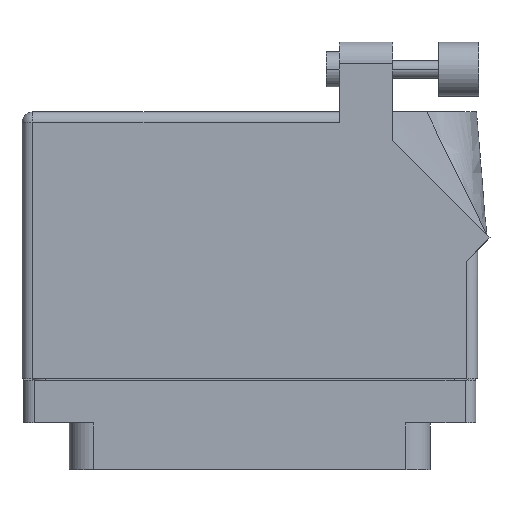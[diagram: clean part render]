
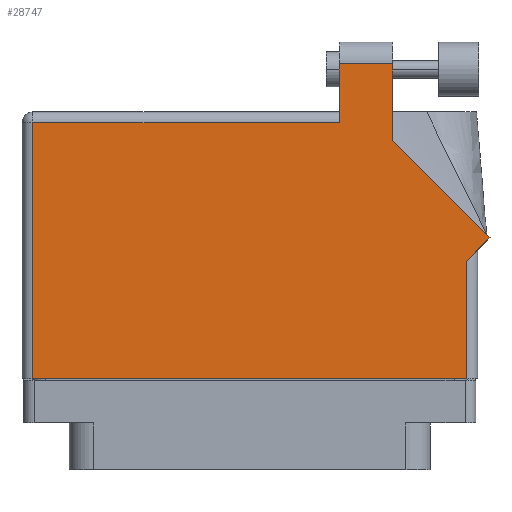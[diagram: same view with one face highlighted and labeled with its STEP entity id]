
A CAD part, front view. The second image highlights one B-rep face of the part: STEP entity #28747.
In plain terms, the highlighted face is planar.
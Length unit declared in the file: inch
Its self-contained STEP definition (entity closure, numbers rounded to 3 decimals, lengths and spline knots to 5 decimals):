
#9 = CARTESIAN_POINT ( 'NONE',  ( -1.306, -0.1, 0.455 ) ) ;
#409 = DIRECTION ( 'NONE',  ( 0., 0., -1. ) ) ;
#1162 = CARTESIAN_POINT ( 'NONE',  ( 1.37671, 0.70771, 0.455 ) ) ;
#1805 = EDGE_CURVE ( 'NONE', #40076, #41135, #41123, .T. ) ;
#1938 = LINE ( 'NONE', #38785, #34554 ) ;
#2650 = ORIENTED_EDGE ( 'NONE', *, *, #43815, .T. ) ;
#3377 = DIRECTION ( 'NONE',  ( -1., 0., 0. ) ) ;
#4816 = EDGE_CURVE ( 'NONE', #47818, #17974, #12187, .T. ) ;
#4828 = EDGE_CURVE ( 'NONE', #51017, #42544, #13381, .T. ) ;
#5143 = CARTESIAN_POINT ( 'NONE',  ( -1.306, 1.43, 0.455 ) ) ;
#5159 = LINE ( 'NONE', #15454, #8283 ) ;
#5259 = VECTOR ( 'NONE', #15422, 39.37008 ) ;
#7045 = CARTESIAN_POINT ( 'NONE',  ( 0.513, 1.705, 0.455 ) ) ;
#7877 = CARTESIAN_POINT ( 'NONE',  ( 0.82, 1.26442, 0.455 ) ) ;
#7932 = ORIENTED_EDGE ( 'NONE', *, *, #10526, .T. ) ;
#8283 = VECTOR ( 'NONE', #3377, 39.37008 ) ;
#10526 = EDGE_CURVE ( 'NONE', #32718, #30651, #5159, .T. ) ;
#11070 = VERTEX_POINT ( 'NONE', #44175 ) ;
#11456 = DIRECTION ( 'NONE',  ( 0., -1., 0. ) ) ;
#11790 = LINE ( 'NONE', #23769, #35677 ) ;
#12187 = LINE ( 'NONE', #9, #34750 ) ;
#12846 = PLANE ( 'NONE',  #20259 ) ;
#13381 = LINE ( 'NONE', #32285, #5259 ) ;
#14507 = DIRECTION ( 'NONE',  ( 0., 1., 0. ) ) ;
#15422 = DIRECTION ( 'NONE',  ( -0.707, 0.707, 0. ) ) ;
#15454 = CARTESIAN_POINT ( 'NONE',  ( 0.513, 1.705, 0.455 ) ) ;
#17049 = LINE ( 'NONE', #35463, #17657 ) ;
#17657 = VECTOR ( 'NONE', #11456, 39.37008 ) ;
#17974 = VERTEX_POINT ( 'NONE', #19095 ) ;
#18078 = ORIENTED_EDGE ( 'NONE', *, *, #4816, .T. ) ;
#19095 = CARTESIAN_POINT ( 'NONE',  ( 1.244, -0.1, 0.455 ) ) ;
#19635 = DIRECTION ( 'NONE',  ( 1., 0., 0. ) ) ;
#19949 = ORIENTED_EDGE ( 'NONE', *, *, #25836, .T. ) ;
#20259 = AXIS2_PLACEMENT_3D ( 'NONE', #5143, #409, #45152 ) ;
#21161 = LINE ( 'NONE', #22234, #22426 ) ;
#22234 = CARTESIAN_POINT ( 'NONE',  ( 1.244, 0.637, 0.455 ) ) ;
#22426 = VECTOR ( 'NONE', #14507, 39.37008 ) ;
#23164 = EDGE_LOOP ( 'NONE', ( #2650, #7932, #44292, #31699, #47061, #18078, #32034, #19949, #40817 ) ) ;
#23464 = DIRECTION ( 'NONE',  ( 0., 1., 0. ) ) ;
#23769 = CARTESIAN_POINT ( 'NONE',  ( 1.306, 0.637, 0.455 ) ) ;
#24046 = CARTESIAN_POINT ( 'NONE',  ( 0.82, 1.705, 0.455 ) ) ;
#24895 = CARTESIAN_POINT ( 'NONE',  ( -1.244, 1.368, 0.455 ) ) ;
#25836 = EDGE_CURVE ( 'NONE', #11070, #51017, #11790, .T. ) ;
#27938 = EDGE_CURVE ( 'NONE', #30651, #40076, #46776, .T. ) ;
#28747 = ADVANCED_FACE ( 'NONE', ( #34705 ), #12846, .F. ) ;
#29072 = EDGE_CURVE ( 'NONE', #41135, #47818, #17049, .T. ) ;
#29401 = CARTESIAN_POINT ( 'NONE',  ( -1.306, 1.368, 0.455 ) ) ;
#29783 = DIRECTION ( 'NONE',  ( 0., -1., 0. ) ) ;
#30651 = VERTEX_POINT ( 'NONE', #7045 ) ;
#31699 = ORIENTED_EDGE ( 'NONE', *, *, #1805, .T. ) ;
#32034 = ORIENTED_EDGE ( 'NONE', *, *, #36484, .T. ) ;
#32285 = CARTESIAN_POINT ( 'NONE',  ( 1.37671, 0.70771, 0.455 ) ) ;
#32302 = VECTOR ( 'NONE', #29783, 39.37008 ) ;
#32718 = VERTEX_POINT ( 'NONE', #24046 ) ;
#32950 = DIRECTION ( 'NONE',  ( -1., 0., 0. ) ) ;
#34554 = VECTOR ( 'NONE', #23464, 39.37008 ) ;
#34705 = FACE_OUTER_BOUND ( 'NONE', #23164, .T. ) ;
#34750 = VECTOR ( 'NONE', #19635, 39.37008 ) ;
#35327 = CARTESIAN_POINT ( 'NONE',  ( -1.244, -0.1, 0.455 ) ) ;
#35463 = CARTESIAN_POINT ( 'NONE',  ( -1.244, -0.1, 0.455 ) ) ;
#35677 = VECTOR ( 'NONE', #47538, 39.37008 ) ;
#36484 = EDGE_CURVE ( 'NONE', #17974, #11070, #21161, .T. ) ;
#38057 = CARTESIAN_POINT ( 'NONE',  ( 0.513, 1.43, 0.455 ) ) ;
#38785 = CARTESIAN_POINT ( 'NONE',  ( 0.82, 1.26442, 0.455 ) ) ;
#40076 = VERTEX_POINT ( 'NONE', #49863 ) ;
#40817 = ORIENTED_EDGE ( 'NONE', *, *, #4828, .T. ) ;
#41123 = LINE ( 'NONE', #29401, #49289 ) ;
#41135 = VERTEX_POINT ( 'NONE', #24895 ) ;
#42544 = VERTEX_POINT ( 'NONE', #7877 ) ;
#43815 = EDGE_CURVE ( 'NONE', #42544, #32718, #1938, .T. ) ;
#44175 = CARTESIAN_POINT ( 'NONE',  ( 1.244, 0.575, 0.455 ) ) ;
#44292 = ORIENTED_EDGE ( 'NONE', *, *, #27938, .T. ) ;
#45152 = DIRECTION ( 'NONE',  ( -1., 0., 0. ) ) ;
#46776 = LINE ( 'NONE', #38057, #32302 ) ;
#47061 = ORIENTED_EDGE ( 'NONE', *, *, #29072, .T. ) ;
#47538 = DIRECTION ( 'NONE',  ( 0.707, 0.707, 0. ) ) ;
#47818 = VERTEX_POINT ( 'NONE', #35327 ) ;
#49289 = VECTOR ( 'NONE', #32950, 39.37008 ) ;
#49863 = CARTESIAN_POINT ( 'NONE',  ( 0.513, 1.368, 0.455 ) ) ;
#51017 = VERTEX_POINT ( 'NONE', #1162 ) ;
